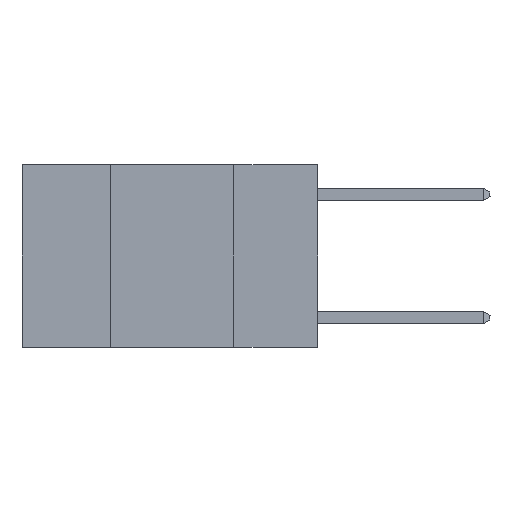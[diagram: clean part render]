
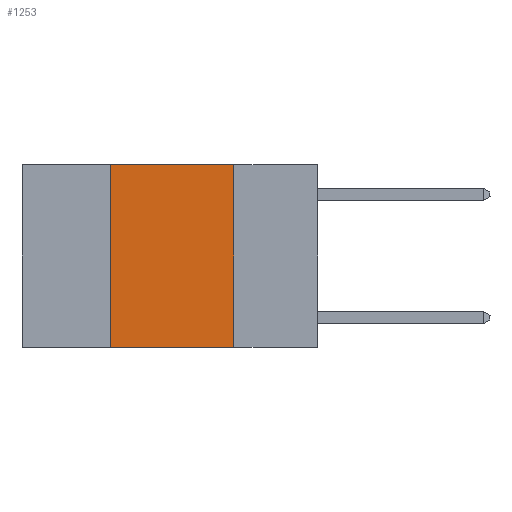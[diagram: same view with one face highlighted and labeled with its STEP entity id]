
A CAD part, left-side view. The second image highlights one B-rep face of the part: STEP entity #1253.
In plain terms, the highlighted planar face has unit normal (-1, 0, 0).
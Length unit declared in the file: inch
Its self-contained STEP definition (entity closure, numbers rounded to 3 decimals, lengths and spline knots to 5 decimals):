
#67 = ORIENTED_EDGE ( 'NONE', *, *, #6363, .F. ) ;
#811 = CARTESIAN_POINT ( 'NONE',  ( 0., 0.17, 0. ) ) ;
#1253 = ADVANCED_FACE ( 'NONE', ( #8023 ), #12325, .F. ) ;
#2032 = EDGE_LOOP ( 'NONE', ( #67, #13614, #14551, #10148 ) ) ;
#2335 = CARTESIAN_POINT ( 'NONE',  ( 0., 0.6, 0. ) ) ;
#3115 = LINE ( 'NONE', #7628, #7765 ) ;
#3323 = EDGE_CURVE ( 'NONE', #4008, #5147, #5865, .T. ) ;
#4008 = VERTEX_POINT ( 'NONE', #12426 ) ;
#4586 = CARTESIAN_POINT ( 'NONE',  ( 0., 0.42, 0. ) ) ;
#5147 = VERTEX_POINT ( 'NONE', #4586 ) ;
#5377 = CARTESIAN_POINT ( 'NONE',  ( 0., 0.6, 0. ) ) ;
#5527 = VECTOR ( 'NONE', #8165, 39.37008 ) ;
#5843 = VERTEX_POINT ( 'NONE', #8028 ) ;
#5865 = LINE ( 'NONE', #13796, #5527 ) ;
#5918 = DIRECTION ( 'NONE',  ( 0., 0., -1. ) ) ;
#6363 = EDGE_CURVE ( 'NONE', #12694, #5843, #12818, .T. ) ;
#7182 = CARTESIAN_POINT ( 'NONE',  ( 0., 0.17, 0. ) ) ;
#7336 = AXIS2_PLACEMENT_3D ( 'NONE', #2335, #11171, #7804 ) ;
#7592 = DIRECTION ( 'NONE',  ( 0., -1., 0. ) ) ;
#7628 = CARTESIAN_POINT ( 'NONE',  ( 0., 0.6, -0.37 ) ) ;
#7765 = VECTOR ( 'NONE', #14227, 39.37008 ) ;
#7804 = DIRECTION ( 'NONE',  ( 0., 0., -1. ) ) ;
#8023 = FACE_OUTER_BOUND ( 'NONE', #2032, .T. ) ;
#8028 = CARTESIAN_POINT ( 'NONE',  ( 0., 0.17, -0.37 ) ) ;
#8165 = DIRECTION ( 'NONE',  ( 0., 0., 1. ) ) ;
#8213 = EDGE_CURVE ( 'NONE', #5147, #12694, #11914, .T. ) ;
#10148 = ORIENTED_EDGE ( 'NONE', *, *, #13380, .T. ) ;
#11171 = DIRECTION ( 'NONE',  ( 1., 0., 0. ) ) ;
#11193 = VECTOR ( 'NONE', #5918, 39.37008 ) ;
#11328 = VECTOR ( 'NONE', #7592, 39.37008 ) ;
#11914 = LINE ( 'NONE', #5377, #11328 ) ;
#12325 = PLANE ( 'NONE',  #7336 ) ;
#12426 = CARTESIAN_POINT ( 'NONE',  ( 0., 0.42, -0.37 ) ) ;
#12694 = VERTEX_POINT ( 'NONE', #811 ) ;
#12818 = LINE ( 'NONE', #7182, #11193 ) ;
#13380 = EDGE_CURVE ( 'NONE', #4008, #5843, #3115, .T. ) ;
#13614 = ORIENTED_EDGE ( 'NONE', *, *, #8213, .F. ) ;
#13796 = CARTESIAN_POINT ( 'NONE',  ( 0., 0.42, 0. ) ) ;
#14227 = DIRECTION ( 'NONE',  ( 0., -1., 0. ) ) ;
#14551 = ORIENTED_EDGE ( 'NONE', *, *, #3323, .F. ) ;
